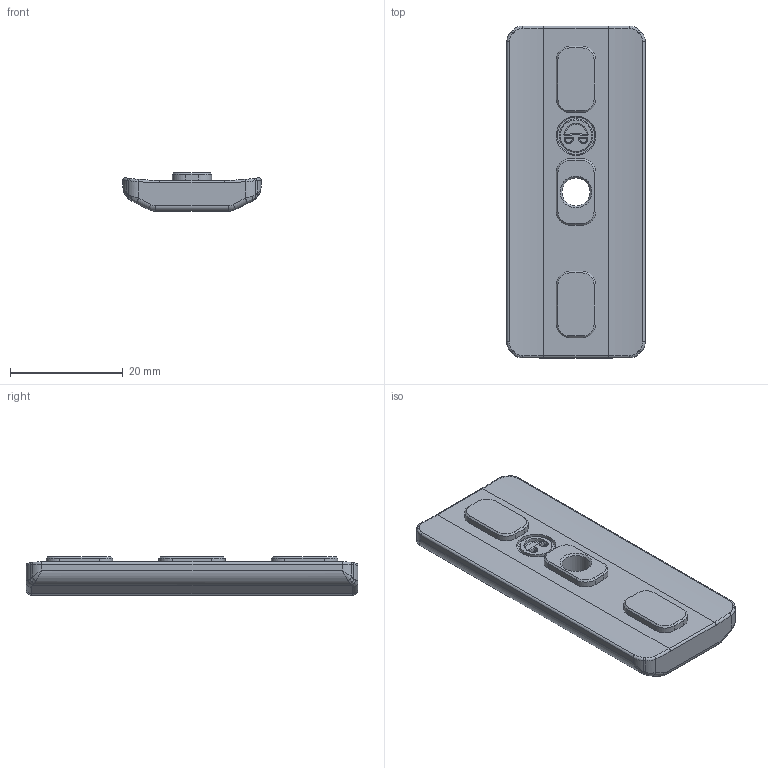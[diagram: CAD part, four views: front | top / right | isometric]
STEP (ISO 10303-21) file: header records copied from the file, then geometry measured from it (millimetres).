
FILE_DESCRIPTION(/* description */ (''),/* implementation_level */ '2;1');
FILE_NAME(/* name */ '1.5 Slot.step',/* time_stamp */ '2021-09-30T11:31:24-04:00',/* author */ (''),/* organization */ (''),/* preprocessor_version */ 'ST-DEVELOPER v18.1',/* originating_system */ 'Autodesk Translation Framework v10.10.0.1391',/* authorisation */ '');
FILE_SCHEMA (('AUTOMOTIVE_DESIGN { 1 0 10303 214 3 1 1 }'));
Length unit declared in the file: millimetre
Products named in the file (1): 1.5 Slot
Bounding box: 24.6 x 59 x 6.85 mm (x, y, z)
Volume: 7228.1 mm3; surface area: 3737.7 mm2
Topology: 1 solids, 1 shells, 161 faces, 367 edges, 213 vertices
Faces by surface type: cylinder 52, plane 45, bspline 30, torus 16, cone 14, sphere 4
Full cylindrical faces by diameter (mm): 5 x1, 5.6 x1, 7 x1, 9.3 x1
Entity records: 5040 total; most frequent: CARTESIAN_POINT 1438, DIRECTION 770, ORIENTED_EDGE 726, EDGE_CURVE 363, AXIS2_PLACEMENT_3D 311, VERTEX_POINT 213, EDGE_LOOP 172, FACE_OUTER_BOUND 161
